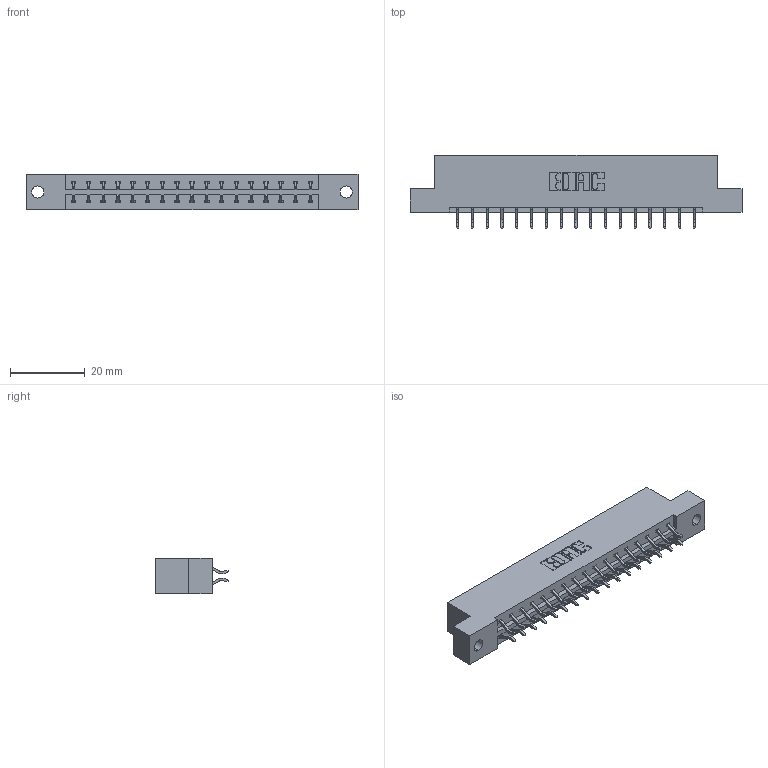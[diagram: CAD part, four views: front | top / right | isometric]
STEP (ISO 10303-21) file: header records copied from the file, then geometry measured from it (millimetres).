
FILE_DESCRIPTION (( 'STEP AP203' ), '1' );
FILE_NAME ('333-034-556-202.STEP', '2018-08-02T22:49:11', ( '' ), ( '' ), 'SwSTEP 2.0', 'SolidWorks 2016', '' );
FILE_SCHEMA (( 'CONFIG_CONTROL_DESIGN' ));
Length unit declared in the file: inch
Products named in the file (3): 333-034-556-202; 333 Part_Flush - .128 Dia; 345-292-001_556 Tail
Assembly tree (35 placements, depth 2):
  333-034-556-202
    333 Part_Flush - .128 Dia
    345-292-001_556 Tail  x34
Bounding box: 88.9 x 19.57 x 9.4 mm (x, y, z)
Volume: 8804.4 mm3; surface area: 9833.4 mm2
Topology: 35 solids, 35 shells, 2086 faces, 6193 edges, 4082 vertices
Faces by surface type: plane 1430, cylinder 656
Entity records: 14393 total; most frequent: CARTESIAN_POINT 2430, ORIENTED_EDGE 2354, DIRECTION 2109, EDGE_CURVE 1177, VECTOR 1041, LINE 1041, VERTEX_POINT 782, AXIS2_PLACEMENT_3D 534
